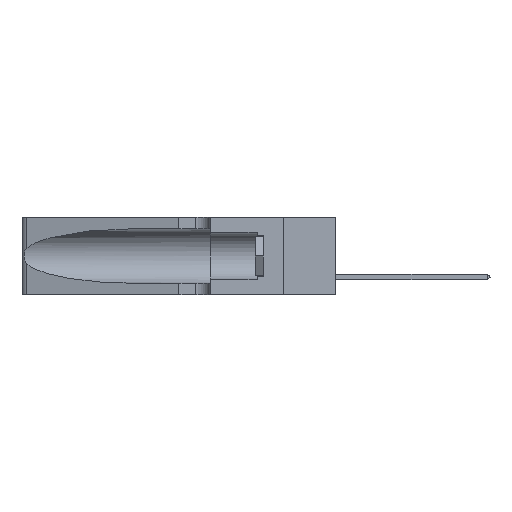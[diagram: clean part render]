
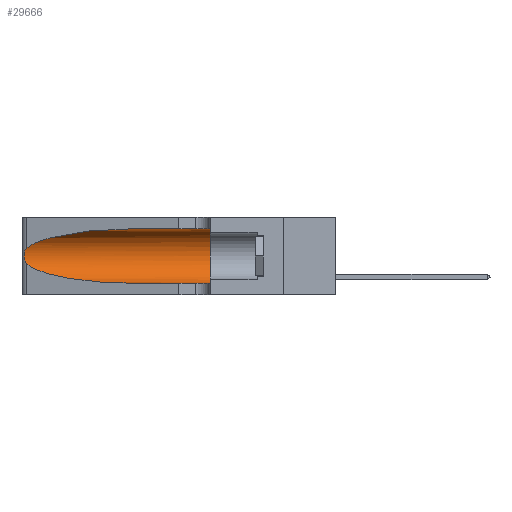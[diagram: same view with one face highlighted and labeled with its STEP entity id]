
A CAD part, left-side view. The second image highlights one B-rep face of the part: STEP entity #29666.
In plain terms, the highlighted cylindrical face has radius 3.308 mm (diameter 6.617 mm), a partial arc.
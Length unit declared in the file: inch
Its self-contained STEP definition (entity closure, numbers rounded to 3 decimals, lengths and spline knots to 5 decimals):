
#66 = CARTESIAN_POINT ( 'NONE',  ( 0.25854, 1.2359, 0.20912 ) ) ;
#833 = CARTESIAN_POINT ( 'NONE',  ( 0.25487, 1.22718, 0.14631 ) ) ;
#1050 = CARTESIAN_POINT ( 'NONE',  ( 0.1305, 1.61858, 0.05475 ) ) ;
#1166 = VERTEX_POINT ( 'NONE', #26299 ) ;
#4124 = CARTESIAN_POINT ( 'NONE',  ( 0.26017, 1.23833, 0.17102 ) ) ;
#5707 = EDGE_CURVE ( 'NONE', #1166, #6572, #33190, .T. ) ;
#6572 = VERTEX_POINT ( 'NONE', #44587 ) ;
#7559 = CARTESIAN_POINT ( 'NONE',  ( 0.25487, 1.22718, 0.22369 ) ) ;
#7765 = DIRECTION ( 'NONE',  ( 0., -1., 0. ) ) ;
#8085 = EDGE_CURVE ( 'NONE', #6572, #44082, #43348, .T. ) ;
#8330 = VERTEX_POINT ( 'NONE', #30091 ) ;
#9916 = CARTESIAN_POINT ( 'NONE',  ( 0.2373, 1.15595, 0.28018 ) ) ;
#12142 = CARTESIAN_POINT ( 'NONE',  ( 0.25555, 1.22993, 0.14849 ) ) ;
#12627 = CARTESIAN_POINT ( 'NONE',  ( 0.1305, 0.35, 0.185 ) ) ;
#12869 = LINE ( 'NONE', #41632, #14710 ) ;
#14019 = CARTESIAN_POINT ( 'NONE',  ( 0.1305, 0.72297, 0.31525 ) ) ;
#14474 = ORIENTED_EDGE ( 'NONE', *, *, #8085, .T. ) ;
#14710 = VECTOR ( 'NONE', #15062, 39.37008 ) ;
#14832 = CARTESIAN_POINT ( 'NONE',  ( 0.25555, 1.22994, 0.2215 ) ) ;
#15062 = DIRECTION ( 'NONE',  ( 0., -1., 0. ) ) ;
#15377 = CARTESIAN_POINT ( 'NONE',  ( 0.18966, 0.96281, 0.05475 ) ) ;
#15648 = ORIENTED_EDGE ( 'NONE', *, *, #16046, .T. ) ;
#16046 = EDGE_CURVE ( 'NONE', #23416, #1166, #31954, .T. ) ;
#16522 = FACE_OUTER_BOUND ( 'NONE', #38430, .T. ) ;
#17492 = CARTESIAN_POINT ( 'NONE',  ( 0.25487, 1.22718, 0.22369 ) ) ;
#19008 = CARTESIAN_POINT ( 'NONE',  ( 0.2373, 1.15595, 0.08982 ) ) ;
#19091 = CARTESIAN_POINT ( 'NONE',  ( 0.25639, 1.23186, 0.15144 ) ) ;
#19381 = EDGE_CURVE ( 'NONE', #44082, #39283, #43598, .T. ) ;
#19737 = CARTESIAN_POINT ( 'NONE',  ( 0.26075, 1.23896, 0.178 ) ) ;
#19769 = DIRECTION ( 'NONE',  ( 0., 0., -1. ) ) ;
#20248 = DIRECTION ( 'NONE',  ( 0., 1., 0. ) ) ;
#22417 = CARTESIAN_POINT ( 'NONE',  ( 0.25787, 1.23484, 0.2124 ) ) ;
#22861 = EDGE_CURVE ( 'NONE', #23416, #8330, #12869, .T. ) ;
#23202 = CARTESIAN_POINT ( 'NONE',  ( 0.1305, 0.35, 0.05475 ) ) ;
#23416 = VERTEX_POINT ( 'NONE', #29772 ) ;
#24237 = VECTOR ( 'NONE', #7765, 39.37008 ) ;
#25766 = ORIENTED_EDGE ( 'NONE', *, *, #22861, .F. ) ;
#26143 = ORIENTED_EDGE ( 'NONE', *, *, #29105, .F. ) ;
#26299 = CARTESIAN_POINT ( 'NONE',  ( 0.25487, 1.22718, 0.22369 ) ) ;
#26807 = CARTESIAN_POINT ( 'NONE',  ( 0.26018, 1.23835, 0.19895 ) ) ;
#27006 = CARTESIAN_POINT ( 'NONE',  ( 0.1305, 1.61858, 0.185 ) ) ;
#29105 = EDGE_CURVE ( 'NONE', #8330, #39283, #47079, .T. ) ;
#29666 = ADVANCED_FACE ( 'NONE', ( #16522 ), #41221, .F. ) ;
#29772 = CARTESIAN_POINT ( 'NONE',  ( 0.1305, 0.72297, 0.31525 ) ) ;
#30091 = CARTESIAN_POINT ( 'NONE',  ( 0.1305, 0.35, 0.31525 ) ) ;
#30195 = CARTESIAN_POINT ( 'NONE',  ( 0.25487, 1.22718, 0.14631 ) ) ;
#31954 =( BOUNDED_CURVE ( )  B_SPLINE_CURVE ( 3, ( #14019, #44367, #9916, #17492 ),
 .UNSPECIFIED., .F., .T. ) 
 B_SPLINE_CURVE_WITH_KNOTS ( ( 4, 4 ),
 ( 1.5708, 2.84003 ),
 .UNSPECIFIED. ) 
 CURVE ( )  GEOMETRIC_REPRESENTATION_ITEM ( )  RATIONAL_B_SPLINE_CURVE ( ( 1., 0.87, 0.87, 1. ) ) 
 REPRESENTATION_ITEM ( '' )  );
#33190 = B_SPLINE_CURVE_WITH_KNOTS ( 'NONE', 3,
 ( #7559, #14832, #48631, #22417, #66, #26807, #34025, #19737, #4124, #38415, #45461, #19091, #12142, #833 ),
 .UNSPECIFIED., .F., .F.,
 ( 4, 2, 2, 2, 2, 2, 4 ),
 ( 0., 0.00027, 0.00053, 0.00107, 0.0016, 0.00187, 0.00214 ),
 .UNSPECIFIED. ) ;
#34025 = CARTESIAN_POINT ( 'NONE',  ( 0.26075, 1.23896, 0.19203 ) ) ;
#35810 = CARTESIAN_POINT ( 'NONE',  ( 0.1305, 0.72297, 0.05475 ) ) ;
#38415 = CARTESIAN_POINT ( 'NONE',  ( 0.25856, 1.23593, 0.16098 ) ) ;
#38430 = EDGE_LOOP ( 'NONE', ( #15648, #38523, #14474, #47736, #26143, #25766 ) ) ;
#38523 = ORIENTED_EDGE ( 'NONE', *, *, #5707, .T. ) ;
#39283 = VERTEX_POINT ( 'NONE', #23202 ) ;
#41221 = CYLINDRICAL_SURFACE ( 'NONE', #48245, 0.13025 ) ;
#41625 = AXIS2_PLACEMENT_3D ( 'NONE', #12627, #20248, #43313 ) ;
#41632 = CARTESIAN_POINT ( 'NONE',  ( 0.1305, 1.61858, 0.31525 ) ) ;
#43313 = DIRECTION ( 'NONE',  ( 0., 0., 1. ) ) ;
#43348 =( BOUNDED_CURVE ( )  B_SPLINE_CURVE ( 3, ( #30195, #19008, #15377, #44588 ),
 .UNSPECIFIED., .F., .F. ) 
 B_SPLINE_CURVE_WITH_KNOTS ( ( 4, 4 ),
 ( 3.44316, 4.71239 ),
 .UNSPECIFIED. ) 
 CURVE ( )  GEOMETRIC_REPRESENTATION_ITEM ( )  RATIONAL_B_SPLINE_CURVE ( ( 1., 0.87, 0.87, 1. ) ) 
 REPRESENTATION_ITEM ( '' )  );
#43598 = LINE ( 'NONE', #1050, #24237 ) ;
#44082 = VERTEX_POINT ( 'NONE', #35810 ) ;
#44367 = CARTESIAN_POINT ( 'NONE',  ( 0.18966, 0.96281, 0.31525 ) ) ;
#44587 = CARTESIAN_POINT ( 'NONE',  ( 0.25487, 1.22718, 0.14631 ) ) ;
#44588 = CARTESIAN_POINT ( 'NONE',  ( 0.1305, 0.72297, 0.05475 ) ) ;
#45461 = CARTESIAN_POINT ( 'NONE',  ( 0.25789, 1.23486, 0.15765 ) ) ;
#45790 = DIRECTION ( 'NONE',  ( 0., -1., 0. ) ) ;
#47079 = CIRCLE ( 'NONE', #41625, 0.13025 ) ;
#47736 = ORIENTED_EDGE ( 'NONE', *, *, #19381, .T. ) ;
#48245 = AXIS2_PLACEMENT_3D ( 'NONE', #27006, #45790, #19769 ) ;
#48631 = CARTESIAN_POINT ( 'NONE',  ( 0.25639, 1.23184, 0.21858 ) ) ;
